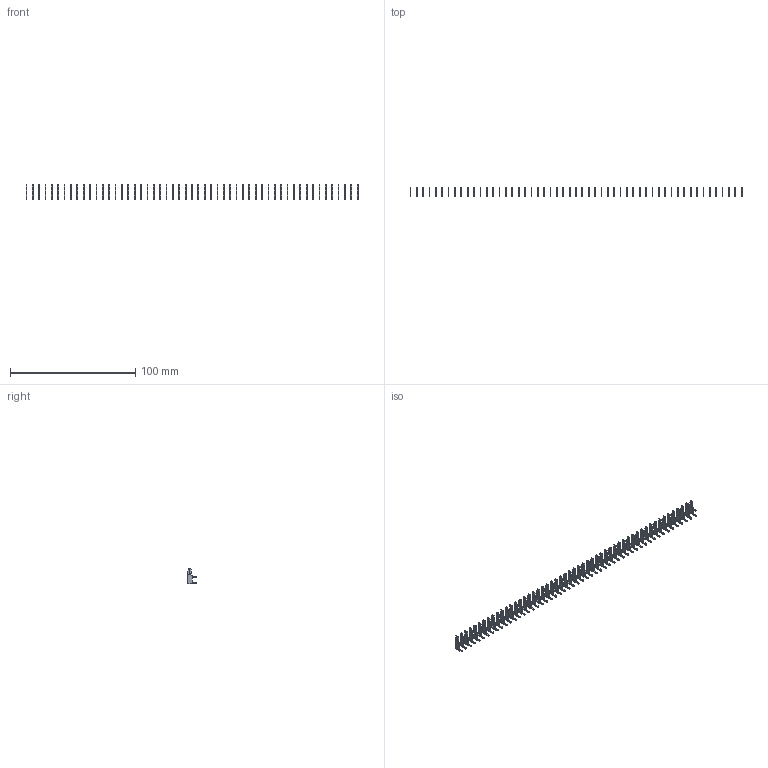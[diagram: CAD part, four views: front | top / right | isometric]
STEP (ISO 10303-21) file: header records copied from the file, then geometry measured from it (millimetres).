
FILE_DESCRIPTION (( 'STEP AP203' ), '1' );
FILE_NAME ('105-053-203-200.STEP', '2020-08-30T00:32:12', ( '' ), ( '' ), 'SwSTEP 2.0', 'SolidWorks 2020', '' );
FILE_SCHEMA (( 'CONFIG_CONTROL_DESIGN' ));
Length unit declared in the file: inch
Products named in the file (2): 100-290-001_100-290-203; 105-053-203-200
Assembly tree (53 placements, depth 2):
  105-053-203-200
    100-290-001_100-290-203  x53
Bounding box: 264.76 x 6.53 x 12.7 mm (x, y, z)
Volume: 1338 mm3; surface area: 6133.1 mm2
Topology: 53 solids, 53 shells, 1484 faces, 4134 edges, 2756 vertices
Faces by surface type: plane 1113, cylinder 371
Entity records: 2760 total; most frequent: DIRECTION 256, CARTESIAN_POINT 226, ORIENTED_EDGE 156, LOCAL_TIME 116, DATE_AND_TIME 116, COORDINATED_UNIVERSAL_TIME_OFFSET 116, CALENDAR_DATE 116, AXIS2_PLACEMENT_3D 98
